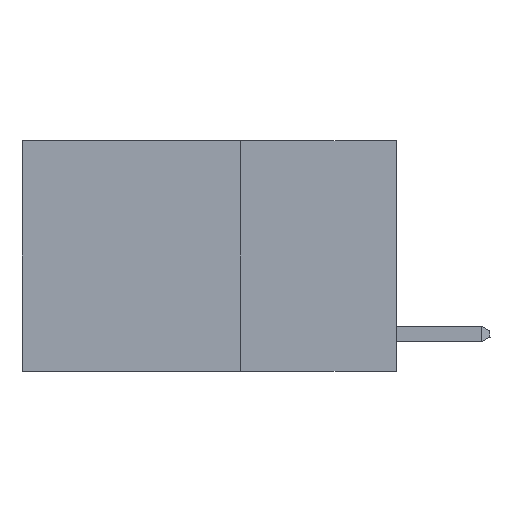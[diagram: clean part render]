
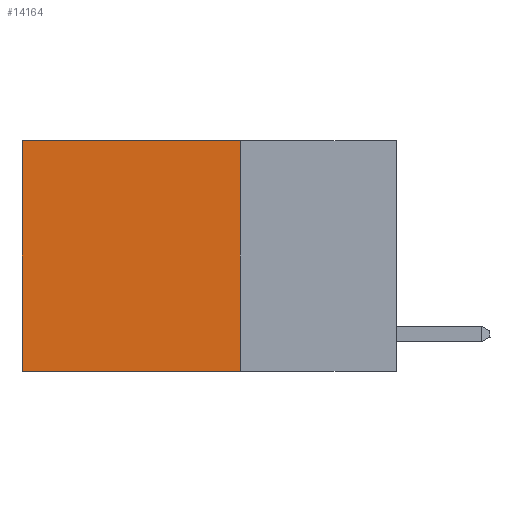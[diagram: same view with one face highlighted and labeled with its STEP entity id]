
A CAD part, left-side view. The second image highlights one B-rep face of the part: STEP entity #14164.
In plain terms, the highlighted planar face has unit normal (-1, 0, 0).
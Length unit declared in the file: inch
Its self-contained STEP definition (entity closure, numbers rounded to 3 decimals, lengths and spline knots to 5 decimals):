
#981 = DIRECTION ( 'NONE',  ( 0., 0., -1. ) ) ;
#1557 = VECTOR ( 'NONE', #981, 39.37008 ) ;
#1571 = CARTESIAN_POINT ( 'NONE',  ( 0.2625, 0.6, 0. ) ) ;
#2102 = VERTEX_POINT ( 'NONE', #15099 ) ;
#3608 = VECTOR ( 'NONE', #7434, 39.37008 ) ;
#3739 = DIRECTION ( 'NONE',  ( 0., 1., 0. ) ) ;
#3784 = LINE ( 'NONE', #11803, #20922 ) ;
#3812 = DIRECTION ( 'NONE',  ( 0., 1., 0. ) ) ;
#4969 = EDGE_CURVE ( 'NONE', #19302, #2102, #14796, .T. ) ;
#5441 = CARTESIAN_POINT ( 'NONE',  ( 0.2625, 0.25, -0.37 ) ) ;
#5594 = CARTESIAN_POINT ( 'NONE',  ( 0.2625, 0.25, 0. ) ) ;
#5863 = LINE ( 'NONE', #15479, #1557 ) ;
#5908 = ORIENTED_EDGE ( 'NONE', *, *, #19142, .T. ) ;
#5949 = CARTESIAN_POINT ( 'NONE',  ( 0.2625, 0.25, 0. ) ) ;
#6022 = VERTEX_POINT ( 'NONE', #1571 ) ;
#7338 = EDGE_LOOP ( 'NONE', ( #10155, #12976, #15055, #5908 ) ) ;
#7434 = DIRECTION ( 'NONE',  ( 0., 0., -1. ) ) ;
#7915 = LINE ( 'NONE', #12227, #3608 ) ;
#8868 = DIRECTION ( 'NONE',  ( 0., 0., -1. ) ) ;
#10155 = ORIENTED_EDGE ( 'NONE', *, *, #16752, .T. ) ;
#10606 = CARTESIAN_POINT ( 'NONE',  ( 0.2625, 0.25, -0.37 ) ) ;
#11027 = VECTOR ( 'NONE', #3812, 39.37008 ) ;
#11543 = FACE_OUTER_BOUND ( 'NONE', #7338, .T. ) ;
#11803 = CARTESIAN_POINT ( 'NONE',  ( 0.2625, 0.25, 0. ) ) ;
#12227 = CARTESIAN_POINT ( 'NONE',  ( 0.2625, 0.25, 0. ) ) ;
#12976 = ORIENTED_EDGE ( 'NONE', *, *, #4969, .F. ) ;
#14164 = ADVANCED_FACE ( 'NONE', ( #11543 ), #20038, .F. ) ;
#14796 = LINE ( 'NONE', #5441, #11027 ) ;
#15055 = ORIENTED_EDGE ( 'NONE', *, *, #16169, .F. ) ;
#15099 = CARTESIAN_POINT ( 'NONE',  ( 0.2625, 0.6, -0.37 ) ) ;
#15479 = CARTESIAN_POINT ( 'NONE',  ( 0.2625, 0.6, 0. ) ) ;
#16169 = EDGE_CURVE ( 'NONE', #20319, #19302, #7915, .T. ) ;
#16752 = EDGE_CURVE ( 'NONE', #6022, #2102, #5863, .T. ) ;
#17023 = AXIS2_PLACEMENT_3D ( 'NONE', #5594, #18510, #8868 ) ;
#18510 = DIRECTION ( 'NONE',  ( 1., 0., 0. ) ) ;
#19142 = EDGE_CURVE ( 'NONE', #20319, #6022, #3784, .T. ) ;
#19302 = VERTEX_POINT ( 'NONE', #10606 ) ;
#20038 = PLANE ( 'NONE',  #17023 ) ;
#20319 = VERTEX_POINT ( 'NONE', #5949 ) ;
#20922 = VECTOR ( 'NONE', #3739, 39.37008 ) ;
